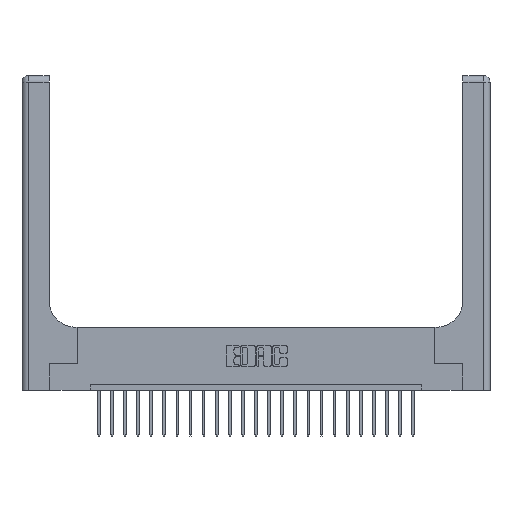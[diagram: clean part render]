
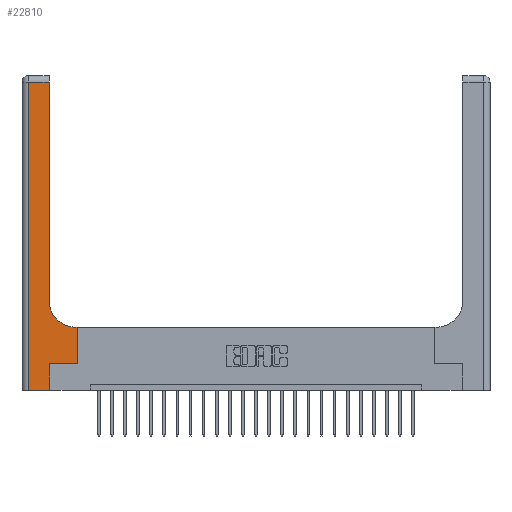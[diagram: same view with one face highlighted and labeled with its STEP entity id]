
A CAD part, top view. The second image highlights one B-rep face of the part: STEP entity #22810.
In plain terms, the highlighted planar face has unit normal (0, 0, 1).
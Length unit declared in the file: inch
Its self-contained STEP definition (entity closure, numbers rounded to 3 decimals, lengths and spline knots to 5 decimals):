
#53 = AXIS2_PLACEMENT_3D ( 'NONE', #4640, #2859, #20699 ) ;
#692 = VERTEX_POINT ( 'NONE', #4448 ) ;
#967 = CARTESIAN_POINT ( 'NONE',  ( 0.06, 3., 0.37 ) ) ;
#1301 = ORIENTED_EDGE ( 'NONE', *, *, #5014, .T. ) ;
#2058 = ORIENTED_EDGE ( 'NONE', *, *, #20927, .T. ) ;
#2111 = DIRECTION ( 'NONE',  ( 0., 0., -1. ) ) ;
#2859 = DIRECTION ( 'NONE',  ( 0., 0., -1. ) ) ;
#3287 = LINE ( 'NONE', #18446, #7688 ) ;
#3326 = CARTESIAN_POINT ( 'NONE',  ( 0., 2.94, 0.37 ) ) ;
#3371 = VECTOR ( 'NONE', #12906, 39.37008 ) ;
#3683 = EDGE_LOOP ( 'NONE', ( #5381, #2058, #5905, #7055, #6614, #10867, #19455, #1301, #16129 ) ) ;
#3973 = DIRECTION ( 'NONE',  ( 0., 1., 0. ) ) ;
#4059 = CARTESIAN_POINT ( 'NONE',  ( 0.26, 3., 0.37 ) ) ;
#4448 = CARTESIAN_POINT ( 'NONE',  ( 0.265, 0.25, 0.37 ) ) ;
#4640 = CARTESIAN_POINT ( 'NONE',  ( 0.51, 0.85, 0.37 ) ) ;
#4766 = DIRECTION ( 'NONE',  ( -1., 0., 0. ) ) ;
#4841 = CIRCLE ( 'NONE', #53, 0.25 ) ;
#4983 = VERTEX_POINT ( 'NONE', #6330 ) ;
#5014 = EDGE_CURVE ( 'NONE', #22115, #17963, #16414, .T. ) ;
#5327 = CARTESIAN_POINT ( 'NONE',  ( 0.528, 0.25, 0.37 ) ) ;
#5381 = ORIENTED_EDGE ( 'NONE', *, *, #9160, .T. ) ;
#5728 = DIRECTION ( 'NONE',  ( -1., 0., 0. ) ) ;
#5905 = ORIENTED_EDGE ( 'NONE', *, *, #10427, .T. ) ;
#6011 = DIRECTION ( 'NONE',  ( 0., 1., 0. ) ) ;
#6330 = CARTESIAN_POINT ( 'NONE',  ( 0.06, 0., 0.37 ) ) ;
#6614 = ORIENTED_EDGE ( 'NONE', *, *, #13689, .T. ) ;
#6900 = CARTESIAN_POINT ( 'NONE',  ( 0.26, 0.6, 0.37 ) ) ;
#7055 = ORIENTED_EDGE ( 'NONE', *, *, #8606, .T. ) ;
#7688 = VECTOR ( 'NONE', #6011, 39.37008 ) ;
#8080 = LINE ( 'NONE', #9532, #3371 ) ;
#8188 = VECTOR ( 'NONE', #8436, 39.37008 ) ;
#8426 = EDGE_CURVE ( 'NONE', #17963, #10651, #4841, .T. ) ;
#8436 = DIRECTION ( 'NONE',  ( 1., 0., 0. ) ) ;
#8606 = EDGE_CURVE ( 'NONE', #4983, #15528, #15161, .T. ) ;
#9160 = EDGE_CURVE ( 'NONE', #10651, #22650, #9720, .T. ) ;
#9266 = CARTESIAN_POINT ( 'NONE',  ( 0., 3., 0.37 ) ) ;
#9532 = CARTESIAN_POINT ( 'NONE',  ( 0.265, 0., 0.37 ) ) ;
#9720 = LINE ( 'NONE', #4059, #18017 ) ;
#10124 = EDGE_CURVE ( 'NONE', #12125, #22115, #3287, .T. ) ;
#10427 = EDGE_CURVE ( 'NONE', #19999, #4983, #16059, .T. ) ;
#10651 = VERTEX_POINT ( 'NONE', #19584 ) ;
#10807 = FACE_OUTER_BOUND ( 'NONE', #3683, .T. ) ;
#10867 = ORIENTED_EDGE ( 'NONE', *, *, #15912, .T. ) ;
#12125 = VERTEX_POINT ( 'NONE', #5327 ) ;
#12552 = DIRECTION ( 'NONE',  ( 1., 0., 0. ) ) ;
#12819 = CARTESIAN_POINT ( 'NONE',  ( 0.26, 2.94, 0.37 ) ) ;
#12906 = DIRECTION ( 'NONE',  ( 0., 1., 0. ) ) ;
#13596 = VECTOR ( 'NONE', #15207, 39.37008 ) ;
#13657 = VECTOR ( 'NONE', #4766, 39.37008 ) ;
#13689 = EDGE_CURVE ( 'NONE', #15528, #692, #8080, .T. ) ;
#14674 = LINE ( 'NONE', #19248, #17691 ) ;
#14727 = LINE ( 'NONE', #3326, #13657 ) ;
#15161 = LINE ( 'NONE', #19088, #8188 ) ;
#15207 = DIRECTION ( 'NONE',  ( 0., -1., 0. ) ) ;
#15321 = VECTOR ( 'NONE', #21018, 39.37008 ) ;
#15528 = VERTEX_POINT ( 'NONE', #21089 ) ;
#15828 = CARTESIAN_POINT ( 'NONE',  ( 0.51, 0.6, 0.37 ) ) ;
#15912 = EDGE_CURVE ( 'NONE', #692, #12125, #14674, .T. ) ;
#16059 = LINE ( 'NONE', #967, #13596 ) ;
#16129 = ORIENTED_EDGE ( 'NONE', *, *, #8426, .T. ) ;
#16414 = LINE ( 'NONE', #6900, #15321 ) ;
#17691 = VECTOR ( 'NONE', #12552, 39.37008 ) ;
#17963 = VERTEX_POINT ( 'NONE', #15828 ) ;
#18017 = VECTOR ( 'NONE', #3973, 39.37008 ) ;
#18446 = CARTESIAN_POINT ( 'NONE',  ( 0.528, 0.25, 0.37 ) ) ;
#19088 = CARTESIAN_POINT ( 'NONE',  ( 0., 0., 0.37 ) ) ;
#19248 = CARTESIAN_POINT ( 'NONE',  ( 0.265, 0.25, 0.37 ) ) ;
#19455 = ORIENTED_EDGE ( 'NONE', *, *, #10124, .T. ) ;
#19584 = CARTESIAN_POINT ( 'NONE',  ( 0.26, 0.85, 0.37 ) ) ;
#19999 = VERTEX_POINT ( 'NONE', #21588 ) ;
#20699 = DIRECTION ( 'NONE',  ( 1., 0., 0. ) ) ;
#20927 = EDGE_CURVE ( 'NONE', #22650, #19999, #14727, .T. ) ;
#21018 = DIRECTION ( 'NONE',  ( -1., 0., 0. ) ) ;
#21089 = CARTESIAN_POINT ( 'NONE',  ( 0.265, 0., 0.37 ) ) ;
#21588 = CARTESIAN_POINT ( 'NONE',  ( 0.06, 2.94, 0.37 ) ) ;
#21592 = PLANE ( 'NONE',  #23010 ) ;
#22115 = VERTEX_POINT ( 'NONE', #22313 ) ;
#22313 = CARTESIAN_POINT ( 'NONE',  ( 0.528, 0.6, 0.37 ) ) ;
#22650 = VERTEX_POINT ( 'NONE', #12819 ) ;
#22810 = ADVANCED_FACE ( 'NONE', ( #10807 ), #21592, .F. ) ;
#23010 = AXIS2_PLACEMENT_3D ( 'NONE', #9266, #2111, #5728 ) ;
